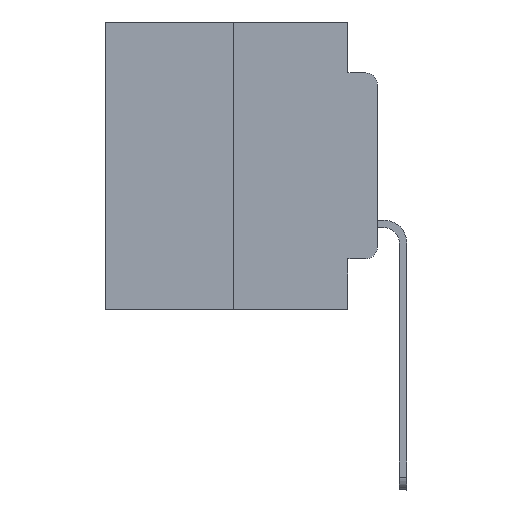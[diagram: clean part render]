
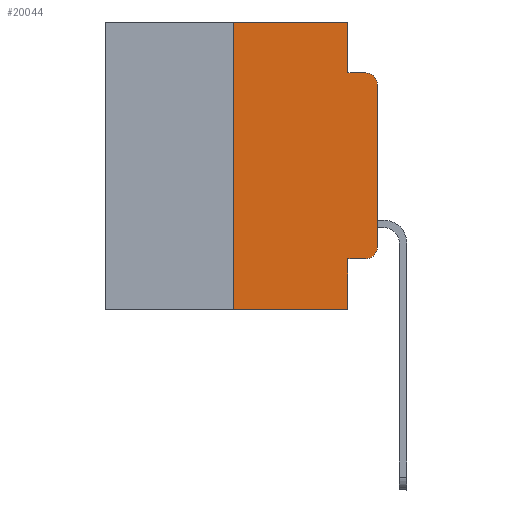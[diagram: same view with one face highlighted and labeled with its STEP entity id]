
A CAD part, left-side view. The second image highlights one B-rep face of the part: STEP entity #20044.
In plain terms, the highlighted planar face has unit normal (-1, 0, 0).
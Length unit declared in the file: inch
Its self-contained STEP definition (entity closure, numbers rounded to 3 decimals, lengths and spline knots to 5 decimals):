
#206 = DIRECTION ( 'NONE',  ( 0., 0., 1. ) ) ;
#398 = CARTESIAN_POINT ( 'NONE',  ( 0., 0.02, -0.1085 ) ) ;
#622 = VERTEX_POINT ( 'NONE', #24461 ) ;
#651 = AXIS2_PLACEMENT_3D ( 'NONE', #16272, #5598, #14155 ) ;
#695 = DIRECTION ( 'NONE',  ( 0., -1., 0. ) ) ;
#964 = EDGE_CURVE ( 'NONE', #26867, #11153, #25960, .T. ) ;
#1597 = AXIS2_PLACEMENT_3D ( 'NONE', #398, #17254, #4067 ) ;
#1599 = CARTESIAN_POINT ( 'NONE',  ( 0., 0.02, -0.4115 ) ) ;
#1959 = VECTOR ( 'NONE', #22224, 39.37008 ) ;
#2300 = CARTESIAN_POINT ( 'NONE',  ( 0., 0.051, 0. ) ) ;
#2425 = CARTESIAN_POINT ( 'NONE',  ( 0., 0.051, 0. ) ) ;
#2441 = DIRECTION ( 'NONE',  ( 0., 0., -1. ) ) ;
#3007 = LINE ( 'NONE', #7217, #24958 ) ;
#3229 = ORIENTED_EDGE ( 'NONE', *, *, #4196, .F. ) ;
#3424 = ORIENTED_EDGE ( 'NONE', *, *, #964, .T. ) ;
#4067 = DIRECTION ( 'NONE',  ( 0., 0., -1. ) ) ;
#4196 = EDGE_CURVE ( 'NONE', #622, #21733, #21971, .T. ) ;
#4395 = CARTESIAN_POINT ( 'NONE',  ( 0., 0.02, -0.3915 ) ) ;
#4424 = EDGE_CURVE ( 'NONE', #18285, #11954, #20626, .T. ) ;
#4457 = VERTEX_POINT ( 'NONE', #17177 ) ;
#5598 = DIRECTION ( 'NONE',  ( 1., 0., 0. ) ) ;
#5907 = EDGE_CURVE ( 'NONE', #6214, #11153, #19709, .T. ) ;
#6214 = VERTEX_POINT ( 'NONE', #8999 ) ;
#7120 = EDGE_CURVE ( 'NONE', #26867, #25822, #10743, .T. ) ;
#7217 = CARTESIAN_POINT ( 'NONE',  ( 0., 0.051, -0.4115 ) ) ;
#8158 = VECTOR ( 'NONE', #21757, 39.37008 ) ;
#8198 = DIRECTION ( 'NONE',  ( -1., 0., 0. ) ) ;
#8276 = ORIENTED_EDGE ( 'NONE', *, *, #4424, .T. ) ;
#8406 = ORIENTED_EDGE ( 'NONE', *, *, #10079, .T. ) ;
#8648 = CARTESIAN_POINT ( 'NONE',  ( 0., 0.051, 0. ) ) ;
#8916 = LINE ( 'NONE', #2300, #27381 ) ;
#8999 = CARTESIAN_POINT ( 'NONE',  ( 0., 0.051, -0.4115 ) ) ;
#9054 = ORIENTED_EDGE ( 'NONE', *, *, #23281, .T. ) ;
#10079 = EDGE_CURVE ( 'NONE', #11954, #4457, #23803, .T. ) ;
#10743 = LINE ( 'NONE', #19313, #15958 ) ;
#10881 = CARTESIAN_POINT ( 'NONE',  ( 0., 0., 0. ) ) ;
#11077 = ORIENTED_EDGE ( 'NONE', *, *, #17129, .F. ) ;
#11153 = VERTEX_POINT ( 'NONE', #26670 ) ;
#11178 = DIRECTION ( 'NONE',  ( 0., 0., 1. ) ) ;
#11358 = CARTESIAN_POINT ( 'NONE',  ( 0., 0.473, 0. ) ) ;
#11839 = ORIENTED_EDGE ( 'NONE', *, *, #16662, .F. ) ;
#11954 = VERTEX_POINT ( 'NONE', #20395 ) ;
#13111 = CARTESIAN_POINT ( 'NONE',  ( 0., 0.051, -0.0885 ) ) ;
#13744 = VECTOR ( 'NONE', #206, 39.37008 ) ;
#14155 = DIRECTION ( 'NONE',  ( 0., 0., -1. ) ) ;
#14222 = VERTEX_POINT ( 'NONE', #8648 ) ;
#15958 = VECTOR ( 'NONE', #11178, 39.37008 ) ;
#16109 = ORIENTED_EDGE ( 'NONE', *, *, #7120, .F. ) ;
#16149 = ORIENTED_EDGE ( 'NONE', *, *, #5907, .F. ) ;
#16272 = CARTESIAN_POINT ( 'NONE',  ( 0., 0.473, 0. ) ) ;
#16662 = EDGE_CURVE ( 'NONE', #14222, #622, #8916, .T. ) ;
#17129 = EDGE_CURVE ( 'NONE', #25822, #14222, #23856, .T. ) ;
#17143 = EDGE_LOOP ( 'NONE', ( #8406, #21118, #3229, #11839, #11077, #16109, #3424, #16149, #9054, #8276 ) ) ;
#17177 = CARTESIAN_POINT ( 'NONE',  ( 0., 0., -0.1085 ) ) ;
#17254 = DIRECTION ( 'NONE',  ( -1., 0., 0. ) ) ;
#18285 = VERTEX_POINT ( 'NONE', #1599 ) ;
#18379 = FACE_OUTER_BOUND ( 'NONE', #17143, .T. ) ;
#19313 = CARTESIAN_POINT ( 'NONE',  ( 0., 0.25, 0. ) ) ;
#19709 = LINE ( 'NONE', #2425, #1959 ) ;
#19917 = PLANE ( 'NONE',  #651 ) ;
#20044 = ADVANCED_FACE ( 'NONE', ( #18379 ), #19917, .F. ) ;
#20395 = CARTESIAN_POINT ( 'NONE',  ( 0., 0., -0.3915 ) ) ;
#20626 = CIRCLE ( 'NONE', #27341, 0.02 ) ;
#21118 = ORIENTED_EDGE ( 'NONE', *, *, #22222, .T. ) ;
#21459 = CARTESIAN_POINT ( 'NONE',  ( 0., 0.25, -0.5 ) ) ;
#21733 = VERTEX_POINT ( 'NONE', #25021 ) ;
#21757 = DIRECTION ( 'NONE',  ( 0., -1., 0. ) ) ;
#21971 = LINE ( 'NONE', #13111, #26950 ) ;
#22222 = EDGE_CURVE ( 'NONE', #4457, #21733, #26224, .T. ) ;
#22224 = DIRECTION ( 'NONE',  ( 0., 0., -1. ) ) ;
#22440 = CARTESIAN_POINT ( 'NONE',  ( 0., 0.25, 0. ) ) ;
#23281 = EDGE_CURVE ( 'NONE', #6214, #18285, #3007, .T. ) ;
#23476 = DIRECTION ( 'NONE',  ( 0., 0., -1. ) ) ;
#23803 = LINE ( 'NONE', #10881, #13744 ) ;
#23856 = LINE ( 'NONE', #11358, #26061 ) ;
#24291 = CARTESIAN_POINT ( 'NONE',  ( 0., 0.473, -0.5 ) ) ;
#24356 = DIRECTION ( 'NONE',  ( 0., -1., 0. ) ) ;
#24461 = CARTESIAN_POINT ( 'NONE',  ( 0., 0.051, -0.0885 ) ) ;
#24958 = VECTOR ( 'NONE', #25879, 39.37008 ) ;
#25021 = CARTESIAN_POINT ( 'NONE',  ( 0., 0.02, -0.0885 ) ) ;
#25822 = VERTEX_POINT ( 'NONE', #22440 ) ;
#25879 = DIRECTION ( 'NONE',  ( 0., -1., 0. ) ) ;
#25960 = LINE ( 'NONE', #24291, #8158 ) ;
#26061 = VECTOR ( 'NONE', #695, 39.37008 ) ;
#26224 = CIRCLE ( 'NONE', #1597, 0.02 ) ;
#26670 = CARTESIAN_POINT ( 'NONE',  ( 0., 0.051, -0.5 ) ) ;
#26867 = VERTEX_POINT ( 'NONE', #21459 ) ;
#26950 = VECTOR ( 'NONE', #24356, 39.37008 ) ;
#27341 = AXIS2_PLACEMENT_3D ( 'NONE', #4395, #8198, #23476 ) ;
#27381 = VECTOR ( 'NONE', #2441, 39.37008 ) ;
